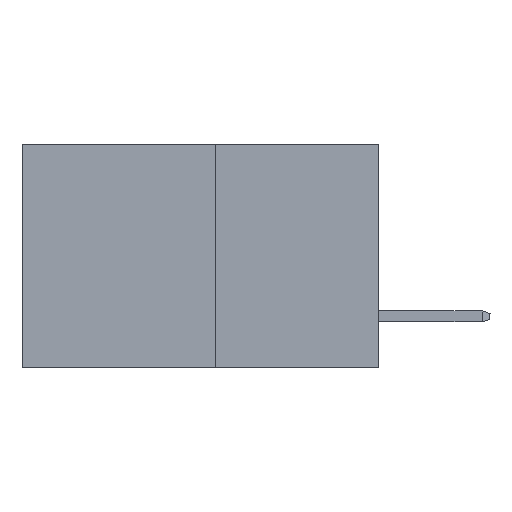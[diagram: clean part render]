
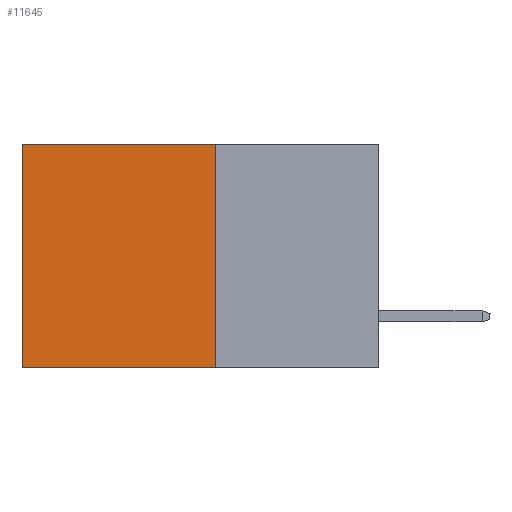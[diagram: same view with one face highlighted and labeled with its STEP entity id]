
A CAD part, left-side view. The second image highlights one B-rep face of the part: STEP entity #11645.
In plain terms, the highlighted planar face has unit normal (-1, 0, 0).
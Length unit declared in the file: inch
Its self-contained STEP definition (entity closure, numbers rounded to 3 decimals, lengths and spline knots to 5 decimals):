
#504 = CARTESIAN_POINT ( 'NONE',  ( 0.277, 0.59, -0.37 ) ) ;
#1040 = LINE ( 'NONE', #5767, #3923 ) ;
#1231 = CARTESIAN_POINT ( 'NONE',  ( 0.277, 0.59, 0. ) ) ;
#1388 = FACE_OUTER_BOUND ( 'NONE', #7909, .T. ) ;
#1396 = DIRECTION ( 'NONE',  ( 0., 0., -1. ) ) ;
#1737 = EDGE_CURVE ( 'NONE', #2941, #8284, #6713, .T. ) ;
#2085 = VECTOR ( 'NONE', #7993, 39.37008 ) ;
#2687 = CARTESIAN_POINT ( 'NONE',  ( 0.277, 0.27, -0.37 ) ) ;
#2941 = VERTEX_POINT ( 'NONE', #1231 ) ;
#3246 = ORIENTED_EDGE ( 'NONE', *, *, #5923, .F. ) ;
#3606 = VECTOR ( 'NONE', #6172, 39.37008 ) ;
#3614 = VERTEX_POINT ( 'NONE', #3970 ) ;
#3923 = VECTOR ( 'NONE', #5959, 39.37008 ) ;
#3970 = CARTESIAN_POINT ( 'NONE',  ( 0.277, 0.27, -0.37 ) ) ;
#4347 = CARTESIAN_POINT ( 'NONE',  ( 0.277, 0.27, 0. ) ) ;
#4503 = VERTEX_POINT ( 'NONE', #10906 ) ;
#5121 = DIRECTION ( 'NONE',  ( 0., 0., -1. ) ) ;
#5330 = LINE ( 'NONE', #4347, #2085 ) ;
#5767 = CARTESIAN_POINT ( 'NONE',  ( 0.277, 0.27, -0.37 ) ) ;
#5923 = EDGE_CURVE ( 'NONE', #3614, #8284, #1040, .T. ) ;
#5959 = DIRECTION ( 'NONE',  ( 0., 1., 0. ) ) ;
#6172 = DIRECTION ( 'NONE',  ( 0., 0., -1. ) ) ;
#6713 = LINE ( 'NONE', #504, #9504 ) ;
#6852 = ORIENTED_EDGE ( 'NONE', *, *, #8973, .F. ) ;
#7341 = CARTESIAN_POINT ( 'NONE',  ( 0.277, 0.59, -0.37 ) ) ;
#7909 = EDGE_LOOP ( 'NONE', ( #14699, #3246, #6852, #10352 ) ) ;
#7993 = DIRECTION ( 'NONE',  ( 0., 1., 0. ) ) ;
#8284 = VERTEX_POINT ( 'NONE', #7341 ) ;
#8720 = AXIS2_PLACEMENT_3D ( 'NONE', #2687, #12123, #5121 ) ;
#8730 = PLANE ( 'NONE',  #8720 ) ;
#8973 = EDGE_CURVE ( 'NONE', #4503, #3614, #9974, .T. ) ;
#9504 = VECTOR ( 'NONE', #1396, 39.37008 ) ;
#9974 = LINE ( 'NONE', #13103, #3606 ) ;
#10352 = ORIENTED_EDGE ( 'NONE', *, *, #14581, .T. ) ;
#10906 = CARTESIAN_POINT ( 'NONE',  ( 0.277, 0.27, 0. ) ) ;
#11645 = ADVANCED_FACE ( 'NONE', ( #1388 ), #8730, .F. ) ;
#12123 = DIRECTION ( 'NONE',  ( 1., 0., 0. ) ) ;
#13103 = CARTESIAN_POINT ( 'NONE',  ( 0.277, 0.27, -0.37 ) ) ;
#14581 = EDGE_CURVE ( 'NONE', #4503, #2941, #5330, .T. ) ;
#14699 = ORIENTED_EDGE ( 'NONE', *, *, #1737, .T. ) ;
